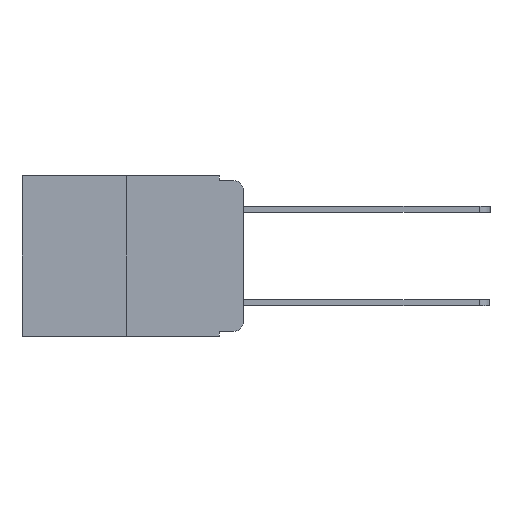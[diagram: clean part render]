
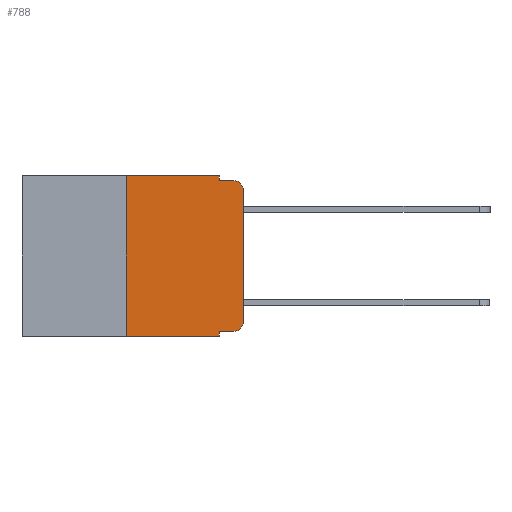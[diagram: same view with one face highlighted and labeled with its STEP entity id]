
A CAD part, left-side view. The second image highlights one B-rep face of the part: STEP entity #788.
In plain terms, the highlighted planar face has unit normal (-1, 0, 0).
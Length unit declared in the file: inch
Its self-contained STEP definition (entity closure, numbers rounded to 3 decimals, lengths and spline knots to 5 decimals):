
#130 = EDGE_LOOP ( 'NONE', ( #2317, #11286, #7126, #11763, #5318, #18062, #10686, #18305, #7556, #16634 ) ) ;
#138 = DIRECTION ( 'NONE',  ( -1., 0., 0. ) ) ;
#233 = CIRCLE ( 'NONE', #17704, 0.02 ) ;
#400 = VECTOR ( 'NONE', #2451, 39.37008 ) ;
#788 = ADVANCED_FACE ( 'NONE', ( #8391 ), #13883, .F. ) ;
#1343 = LINE ( 'NONE', #13959, #13268 ) ;
#1490 = VECTOR ( 'NONE', #18134, 39.37008 ) ;
#1536 = VECTOR ( 'NONE', #15916, 39.37008 ) ;
#2095 = EDGE_CURVE ( 'NONE', #17963, #12322, #3250, .T. ) ;
#2317 = ORIENTED_EDGE ( 'NONE', *, *, #13953, .T. ) ;
#2451 = DIRECTION ( 'NONE',  ( 0., 0., -1. ) ) ;
#3240 = EDGE_CURVE ( 'NONE', #14876, #16045, #14339, .T. ) ;
#3250 = CIRCLE ( 'NONE', #17453, 0.02 ) ;
#3661 = CARTESIAN_POINT ( 'NONE',  ( 0., 0., -0.03 ) ) ;
#3767 = CARTESIAN_POINT ( 'NONE',  ( 0., 0.25, 0. ) ) ;
#4670 = DIRECTION ( 'NONE',  ( 0., -1., 0. ) ) ;
#4856 = VERTEX_POINT ( 'NONE', #17685 ) ;
#5120 = CARTESIAN_POINT ( 'NONE',  ( 0., 0.02, -0.313 ) ) ;
#5318 = ORIENTED_EDGE ( 'NONE', *, *, #20036, .F. ) ;
#5414 = VECTOR ( 'NONE', #17820, 39.37008 ) ;
#5528 = CARTESIAN_POINT ( 'NONE',  ( 0., 0.25, -0.343 ) ) ;
#5829 = VERTEX_POINT ( 'NONE', #12348 ) ;
#5912 = DIRECTION ( 'NONE',  ( 0., 0., -1. ) ) ;
#6025 = DIRECTION ( 'NONE',  ( 0., 0., -1. ) ) ;
#6496 = EDGE_CURVE ( 'NONE', #12855, #13014, #1343, .T. ) ;
#6727 = LINE ( 'NONE', #12835, #14662 ) ;
#6929 = LINE ( 'NONE', #9717, #1536 ) ;
#6949 = DIRECTION ( 'NONE',  ( 1., 0., 0. ) ) ;
#7126 = ORIENTED_EDGE ( 'NONE', *, *, #8677, .F. ) ;
#7155 = CARTESIAN_POINT ( 'NONE',  ( 0., 0.051, 0. ) ) ;
#7291 = CARTESIAN_POINT ( 'NONE',  ( 0., 0.051, 0. ) ) ;
#7556 = ORIENTED_EDGE ( 'NONE', *, *, #20306, .T. ) ;
#7995 = EDGE_CURVE ( 'NONE', #14876, #13014, #6727, .T. ) ;
#8391 = FACE_OUTER_BOUND ( 'NONE', #130, .T. ) ;
#8677 = EDGE_CURVE ( 'NONE', #4856, #5829, #18309, .T. ) ;
#9717 = CARTESIAN_POINT ( 'NONE',  ( 0., 0., 0. ) ) ;
#9761 = EDGE_CURVE ( 'NONE', #11797, #4856, #12900, .T. ) ;
#9910 = CARTESIAN_POINT ( 'NONE',  ( 0., 0.02, -0.333 ) ) ;
#10012 = CARTESIAN_POINT ( 'NONE',  ( 0., 0.02, -0.03 ) ) ;
#10225 = VECTOR ( 'NONE', #11127, 39.37008 ) ;
#10313 = DIRECTION ( 'NONE',  ( 0., 0., -1. ) ) ;
#10460 = VECTOR ( 'NONE', #4670, 39.37008 ) ;
#10474 = CARTESIAN_POINT ( 'NONE',  ( 0., 0.25, 0. ) ) ;
#10686 = ORIENTED_EDGE ( 'NONE', *, *, #7995, .T. ) ;
#11045 = DIRECTION ( 'NONE',  ( -1., 0., 0. ) ) ;
#11067 = CARTESIAN_POINT ( 'NONE',  ( 0., 0.473, 0. ) ) ;
#11127 = DIRECTION ( 'NONE',  ( 0., -1., 0. ) ) ;
#11257 = CARTESIAN_POINT ( 'NONE',  ( 0., 0.473, 0. ) ) ;
#11286 = ORIENTED_EDGE ( 'NONE', *, *, #12928, .T. ) ;
#11605 = DIRECTION ( 'NONE',  ( 0., 0., -1. ) ) ;
#11763 = ORIENTED_EDGE ( 'NONE', *, *, #9761, .F. ) ;
#11797 = VERTEX_POINT ( 'NONE', #7155 ) ;
#12322 = VERTEX_POINT ( 'NONE', #17702 ) ;
#12339 = VERTEX_POINT ( 'NONE', #3661 ) ;
#12348 = CARTESIAN_POINT ( 'NONE',  ( 0., 0.02, -0.01 ) ) ;
#12835 = CARTESIAN_POINT ( 'NONE',  ( 0., 0.473, -0.343 ) ) ;
#12855 = VERTEX_POINT ( 'NONE', #20435 ) ;
#12900 = LINE ( 'NONE', #7291, #400 ) ;
#12928 = EDGE_CURVE ( 'NONE', #12339, #5829, #233, .T. ) ;
#13014 = VERTEX_POINT ( 'NONE', #13329 ) ;
#13268 = VECTOR ( 'NONE', #6025, 39.37008 ) ;
#13329 = CARTESIAN_POINT ( 'NONE',  ( 0., 0.051, -0.343 ) ) ;
#13883 = PLANE ( 'NONE',  #15960 ) ;
#13953 = EDGE_CURVE ( 'NONE', #12322, #12339, #6929, .T. ) ;
#13959 = CARTESIAN_POINT ( 'NONE',  ( 0., 0.051, 0. ) ) ;
#14339 = LINE ( 'NONE', #10474, #1490 ) ;
#14366 = DIRECTION ( 'NONE',  ( 0., -1., 0. ) ) ;
#14621 = LINE ( 'NONE', #11067, #10460 ) ;
#14662 = VECTOR ( 'NONE', #14366, 39.37008 ) ;
#14801 = CARTESIAN_POINT ( 'NONE',  ( 0., 0.051, -0.333 ) ) ;
#14876 = VERTEX_POINT ( 'NONE', #5528 ) ;
#15916 = DIRECTION ( 'NONE',  ( 0., 0., 1. ) ) ;
#15960 = AXIS2_PLACEMENT_3D ( 'NONE', #11257, #6949, #5912 ) ;
#16045 = VERTEX_POINT ( 'NONE', #3767 ) ;
#16634 = ORIENTED_EDGE ( 'NONE', *, *, #2095, .T. ) ;
#17453 = AXIS2_PLACEMENT_3D ( 'NONE', #5120, #11045, #10313 ) ;
#17685 = CARTESIAN_POINT ( 'NONE',  ( 0., 0.051, -0.01 ) ) ;
#17702 = CARTESIAN_POINT ( 'NONE',  ( 0., 0., -0.313 ) ) ;
#17704 = AXIS2_PLACEMENT_3D ( 'NONE', #10012, #138, #11605 ) ;
#17820 = DIRECTION ( 'NONE',  ( 0., -1., 0. ) ) ;
#17835 = LINE ( 'NONE', #14801, #5414 ) ;
#17963 = VERTEX_POINT ( 'NONE', #9910 ) ;
#18062 = ORIENTED_EDGE ( 'NONE', *, *, #3240, .F. ) ;
#18134 = DIRECTION ( 'NONE',  ( 0., 0., 1. ) ) ;
#18305 = ORIENTED_EDGE ( 'NONE', *, *, #6496, .F. ) ;
#18309 = LINE ( 'NONE', #20170, #10225 ) ;
#20036 = EDGE_CURVE ( 'NONE', #16045, #11797, #14621, .T. ) ;
#20170 = CARTESIAN_POINT ( 'NONE',  ( 0., 0.051, -0.01 ) ) ;
#20306 = EDGE_CURVE ( 'NONE', #12855, #17963, #17835, .T. ) ;
#20435 = CARTESIAN_POINT ( 'NONE',  ( 0., 0.051, -0.333 ) ) ;
